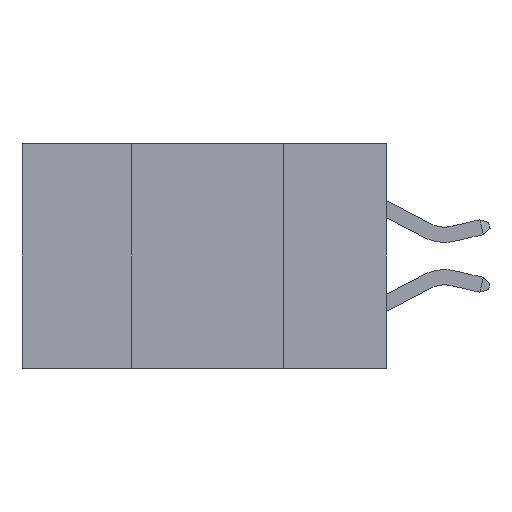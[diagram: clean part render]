
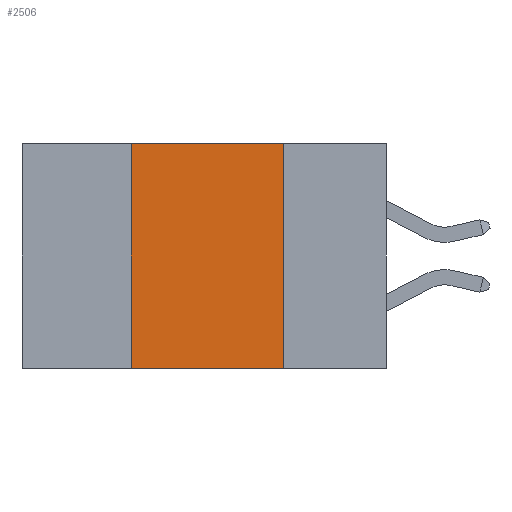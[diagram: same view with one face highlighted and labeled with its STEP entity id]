
A CAD part, left-side view. The second image highlights one B-rep face of the part: STEP entity #2506.
In plain terms, the highlighted planar face has unit normal (-1, 0, 0).
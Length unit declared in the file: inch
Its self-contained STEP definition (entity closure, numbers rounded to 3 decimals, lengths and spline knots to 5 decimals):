
#647 = ORIENTED_EDGE ( 'NONE', *, *, #13189, .T. ) ;
#731 = EDGE_CURVE ( 'NONE', #21484, #13584, #20860, .T. ) ;
#1038 = VERTEX_POINT ( 'NONE', #18038 ) ;
#2506 = ADVANCED_FACE ( 'NONE', ( #9916 ), #16207, .F. ) ;
#2525 = DIRECTION ( 'NONE',  ( 0., -1., 0. ) ) ;
#4381 = VECTOR ( 'NONE', #20460, 39.37008 ) ;
#4691 = CARTESIAN_POINT ( 'NONE',  ( 0., 0.17, -0.37 ) ) ;
#5313 = DIRECTION ( 'NONE',  ( 1., 0., 0. ) ) ;
#5369 = ORIENTED_EDGE ( 'NONE', *, *, #5950, .F. ) ;
#5536 = VECTOR ( 'NONE', #2525, 39.37008 ) ;
#5950 = EDGE_CURVE ( 'NONE', #21704, #1038, #7779, .T. ) ;
#6998 = VECTOR ( 'NONE', #26636, 39.37008 ) ;
#7546 = CARTESIAN_POINT ( 'NONE',  ( 0., 0.17, 0. ) ) ;
#7779 = LINE ( 'NONE', #9598, #6998 ) ;
#8815 = CARTESIAN_POINT ( 'NONE',  ( 0., 0.6, -0.37 ) ) ;
#9503 = CARTESIAN_POINT ( 'NONE',  ( 0., 0.6, 0. ) ) ;
#9598 = CARTESIAN_POINT ( 'NONE',  ( 0., 0.42, -0.37 ) ) ;
#9916 = FACE_OUTER_BOUND ( 'NONE', #12727, .T. ) ;
#10460 = VECTOR ( 'NONE', #16527, 39.37008 ) ;
#11888 = ORIENTED_EDGE ( 'NONE', *, *, #731, .F. ) ;
#12727 = EDGE_LOOP ( 'NONE', ( #11888, #25554, #5369, #647 ) ) ;
#12848 = CARTESIAN_POINT ( 'NONE',  ( 0., 0.42, -0.37 ) ) ;
#13189 = EDGE_CURVE ( 'NONE', #21704, #13584, #17070, .T. ) ;
#13584 = VERTEX_POINT ( 'NONE', #4691 ) ;
#16207 = PLANE ( 'NONE',  #19814 ) ;
#16527 = DIRECTION ( 'NONE',  ( 0., 0., -1. ) ) ;
#16947 = CARTESIAN_POINT ( 'NONE',  ( 0., 0.17, -0.37 ) ) ;
#17070 = LINE ( 'NONE', #8815, #5536 ) ;
#18038 = CARTESIAN_POINT ( 'NONE',  ( 0., 0.42, 0. ) ) ;
#18503 = CARTESIAN_POINT ( 'NONE',  ( 0., 0.6, 0. ) ) ;
#19044 = EDGE_CURVE ( 'NONE', #1038, #21484, #27019, .T. ) ;
#19814 = AXIS2_PLACEMENT_3D ( 'NONE', #9503, #5313, #22206 ) ;
#20460 = DIRECTION ( 'NONE',  ( 0., -1., 0. ) ) ;
#20860 = LINE ( 'NONE', #16947, #10460 ) ;
#21484 = VERTEX_POINT ( 'NONE', #7546 ) ;
#21704 = VERTEX_POINT ( 'NONE', #12848 ) ;
#22206 = DIRECTION ( 'NONE',  ( 0., 0., -1. ) ) ;
#25554 = ORIENTED_EDGE ( 'NONE', *, *, #19044, .F. ) ;
#26636 = DIRECTION ( 'NONE',  ( 0., 0., 1. ) ) ;
#27019 = LINE ( 'NONE', #18503, #4381 ) ;
